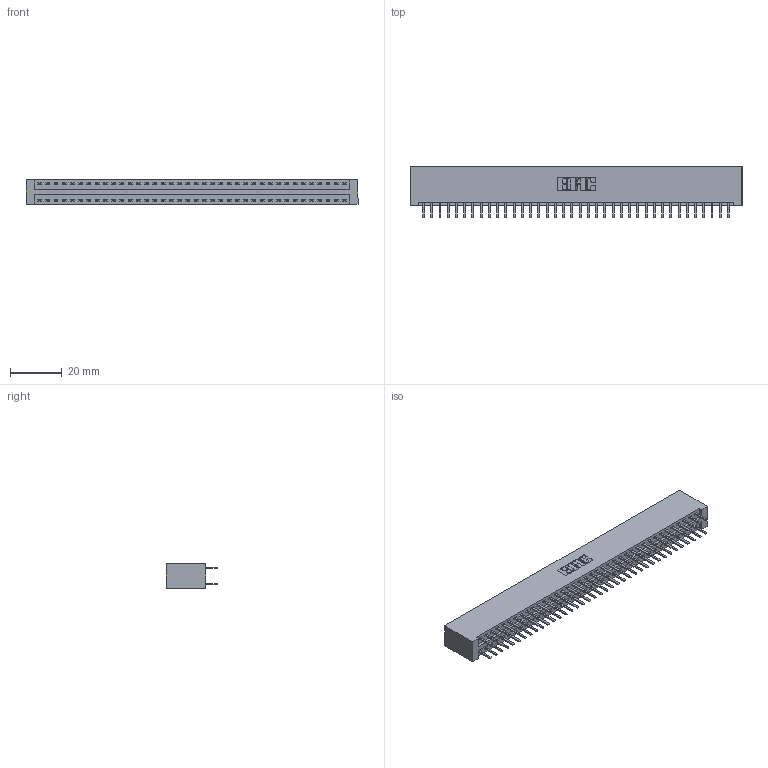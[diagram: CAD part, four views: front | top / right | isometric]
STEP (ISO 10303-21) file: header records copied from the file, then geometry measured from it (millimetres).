
FILE_DESCRIPTION (( 'STEP AP203' ), '1' );
FILE_NAME ('396-076-520-201.STEP', '2019-10-30T21:05:03', ( '' ), ( '' ), 'SwSTEP 2.0', 'SolidWorks 2016', '' );
FILE_SCHEMA (( 'CONFIG_CONTROL_DESIGN' ));
Length unit declared in the file: inch
Products named in the file (3): 346 Part_No Mounting Lugs; 396-076-520-201; 345-292-001_345-293-120
Assembly tree (77 placements, depth 2):
  396-076-520-201
    346 Part_No Mounting Lugs
    345-292-001_345-293-120  x76
Bounding box: 127.89 x 20.02 x 9.4 mm (x, y, z)
Volume: 12979.6 mm3; surface area: 17863.3 mm2
Topology: 77 solids, 77 shells, 4370 faces, 12693 edges, 8258 vertices
Faces by surface type: plane 2884, cylinder 1486
Entity records: 25175 total; most frequent: CARTESIAN_POINT 4164, ORIENTED_EDGE 4086, DIRECTION 3703, EDGE_CURVE 2043, VECTOR 1763, LINE 1763, VERTEX_POINT 1358, AXIS2_PLACEMENT_3D 970
